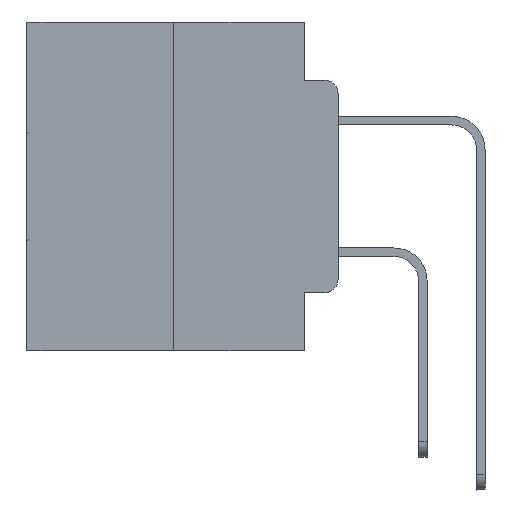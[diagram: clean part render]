
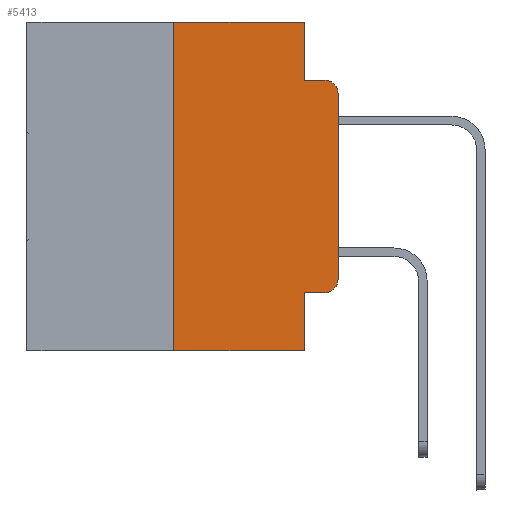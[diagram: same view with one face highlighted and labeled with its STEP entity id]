
A CAD part, left-side view. The second image highlights one B-rep face of the part: STEP entity #5413.
In plain terms, the highlighted planar face has unit normal (-1, 0, 0).
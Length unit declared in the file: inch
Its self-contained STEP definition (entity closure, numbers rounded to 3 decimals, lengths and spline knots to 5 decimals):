
#1445 = EDGE_CURVE ( 'NONE', #25797, #8543, #18991, .T. ) ;
#1482 = ORIENTED_EDGE ( 'NONE', *, *, #1445, .F. ) ;
#1768 = VERTEX_POINT ( 'NONE', #11312 ) ;
#2505 = EDGE_CURVE ( 'NONE', #1768, #14489, #7403, .T. ) ;
#3395 = ORIENTED_EDGE ( 'NONE', *, *, #3486, .T. ) ;
#3486 = EDGE_CURVE ( 'NONE', #14489, #27087, #11125, .T. ) ;
#3939 = VERTEX_POINT ( 'NONE', #16318 ) ;
#4464 = DIRECTION ( 'NONE',  ( 0., -1., 0. ) ) ;
#5152 = LINE ( 'NONE', #9500, #22812 ) ;
#5413 = ADVANCED_FACE ( 'NONE', ( #10085 ), #7814, .F. ) ;
#6423 = ORIENTED_EDGE ( 'NONE', *, *, #21006, .F. ) ;
#7162 = CIRCLE ( 'NONE', #29111, 0.02 ) ;
#7281 = AXIS2_PLACEMENT_3D ( 'NONE', #29395, #24772, #17108 ) ;
#7403 = CIRCLE ( 'NONE', #11485, 0.02 ) ;
#7814 = PLANE ( 'NONE',  #7281 ) ;
#8119 = VECTOR ( 'NONE', #30658, 39.37008 ) ;
#8517 = VECTOR ( 'NONE', #29429, 39.37008 ) ;
#8543 = VERTEX_POINT ( 'NONE', #23139 ) ;
#8775 = ORIENTED_EDGE ( 'NONE', *, *, #24849, .T. ) ;
#9057 = VERTEX_POINT ( 'NONE', #21334 ) ;
#9500 = CARTESIAN_POINT ( 'NONE',  ( 0., 0.051, -0.4115 ) ) ;
#10085 = FACE_OUTER_BOUND ( 'NONE', #21643, .T. ) ;
#10457 = DIRECTION ( 'NONE',  ( 0., 0., -1. ) ) ;
#10911 = EDGE_CURVE ( 'NONE', #23085, #25797, #22246, .T. ) ;
#11125 = LINE ( 'NONE', #16239, #13843 ) ;
#11164 = CARTESIAN_POINT ( 'NONE',  ( 0., 0., -0.1085 ) ) ;
#11312 = CARTESIAN_POINT ( 'NONE',  ( 0., 0.02, -0.4115 ) ) ;
#11485 = AXIS2_PLACEMENT_3D ( 'NONE', #18104, #19876, #10457 ) ;
#11494 = ORIENTED_EDGE ( 'NONE', *, *, #15456, .F. ) ;
#11656 = LINE ( 'NONE', #21563, #8119 ) ;
#12397 = ORIENTED_EDGE ( 'NONE', *, *, #2505, .T. ) ;
#13021 = CARTESIAN_POINT ( 'NONE',  ( 0., 0.25, -0.5 ) ) ;
#13843 = VECTOR ( 'NONE', #25965, 39.37008 ) ;
#14489 = VERTEX_POINT ( 'NONE', #18332 ) ;
#15133 = LINE ( 'NONE', #24864, #30101 ) ;
#15456 = EDGE_CURVE ( 'NONE', #3939, #26605, #11656, .T. ) ;
#16156 = CARTESIAN_POINT ( 'NONE',  ( 0., 0.051, -0.5 ) ) ;
#16172 = EDGE_CURVE ( 'NONE', #23085, #26605, #15133, .T. ) ;
#16239 = CARTESIAN_POINT ( 'NONE',  ( 0., 0., 0. ) ) ;
#16318 = CARTESIAN_POINT ( 'NONE',  ( 0., 0.051, -0.4115 ) ) ;
#16752 = EDGE_CURVE ( 'NONE', #27087, #21633, #7162, .T. ) ;
#16861 = LINE ( 'NONE', #21821, #25201 ) ;
#17108 = DIRECTION ( 'NONE',  ( 0., 0., -1. ) ) ;
#17762 = CARTESIAN_POINT ( 'NONE',  ( 0., 0.25, 0. ) ) ;
#18104 = CARTESIAN_POINT ( 'NONE',  ( 0., 0.02, -0.3915 ) ) ;
#18332 = CARTESIAN_POINT ( 'NONE',  ( 0., 0., -0.3915 ) ) ;
#18660 = DIRECTION ( 'NONE',  ( 0., 0., -1. ) ) ;
#18991 = LINE ( 'NONE', #28741, #31103 ) ;
#19219 = DIRECTION ( 'NONE',  ( 0., -1., 0. ) ) ;
#19876 = DIRECTION ( 'NONE',  ( -1., 0., 0. ) ) ;
#21006 = EDGE_CURVE ( 'NONE', #8543, #9057, #23307, .T. ) ;
#21317 = ORIENTED_EDGE ( 'NONE', *, *, #16172, .T. ) ;
#21334 = CARTESIAN_POINT ( 'NONE',  ( 0., 0.051, -0.0885 ) ) ;
#21362 = ORIENTED_EDGE ( 'NONE', *, *, #29018, .F. ) ;
#21563 = CARTESIAN_POINT ( 'NONE',  ( 0., 0.051, 0. ) ) ;
#21633 = VERTEX_POINT ( 'NONE', #31381 ) ;
#21643 = EDGE_LOOP ( 'NONE', ( #3395, #30545, #21362, #6423, #1482, #23868, #21317, #11494, #8775, #12397 ) ) ;
#21821 = CARTESIAN_POINT ( 'NONE',  ( 0., 0.051, -0.0885 ) ) ;
#22246 = LINE ( 'NONE', #17762, #8517 ) ;
#22812 = VECTOR ( 'NONE', #19219, 39.37008 ) ;
#22915 = DIRECTION ( 'NONE',  ( 0., 0., -1. ) ) ;
#22945 = DIRECTION ( 'NONE',  ( 0., -1., 0. ) ) ;
#23085 = VERTEX_POINT ( 'NONE', #13021 ) ;
#23139 = CARTESIAN_POINT ( 'NONE',  ( 0., 0.051, 0. ) ) ;
#23307 = LINE ( 'NONE', #26005, #24642 ) ;
#23868 = ORIENTED_EDGE ( 'NONE', *, *, #10911, .F. ) ;
#24642 = VECTOR ( 'NONE', #18660, 39.37008 ) ;
#24772 = DIRECTION ( 'NONE',  ( 1., 0., 0. ) ) ;
#24849 = EDGE_CURVE ( 'NONE', #3939, #1768, #5152, .T. ) ;
#24864 = CARTESIAN_POINT ( 'NONE',  ( 0., 0.473, -0.5 ) ) ;
#25201 = VECTOR ( 'NONE', #31542, 39.37008 ) ;
#25797 = VERTEX_POINT ( 'NONE', #27937 ) ;
#25965 = DIRECTION ( 'NONE',  ( 0., 0., 1. ) ) ;
#26005 = CARTESIAN_POINT ( 'NONE',  ( 0., 0.051, 0. ) ) ;
#26206 = DIRECTION ( 'NONE',  ( -1., 0., 0. ) ) ;
#26605 = VERTEX_POINT ( 'NONE', #16156 ) ;
#27087 = VERTEX_POINT ( 'NONE', #11164 ) ;
#27694 = CARTESIAN_POINT ( 'NONE',  ( 0., 0.02, -0.1085 ) ) ;
#27937 = CARTESIAN_POINT ( 'NONE',  ( 0., 0.25, 0. ) ) ;
#28741 = CARTESIAN_POINT ( 'NONE',  ( 0., 0.473, 0. ) ) ;
#29018 = EDGE_CURVE ( 'NONE', #9057, #21633, #16861, .T. ) ;
#29111 = AXIS2_PLACEMENT_3D ( 'NONE', #27694, #26206, #22915 ) ;
#29395 = CARTESIAN_POINT ( 'NONE',  ( 0., 0.473, 0. ) ) ;
#29429 = DIRECTION ( 'NONE',  ( 0., 0., 1. ) ) ;
#30101 = VECTOR ( 'NONE', #22945, 39.37008 ) ;
#30545 = ORIENTED_EDGE ( 'NONE', *, *, #16752, .T. ) ;
#30658 = DIRECTION ( 'NONE',  ( 0., 0., -1. ) ) ;
#31103 = VECTOR ( 'NONE', #4464, 39.37008 ) ;
#31381 = CARTESIAN_POINT ( 'NONE',  ( 0., 0.02, -0.0885 ) ) ;
#31542 = DIRECTION ( 'NONE',  ( 0., -1., 0. ) ) ;
